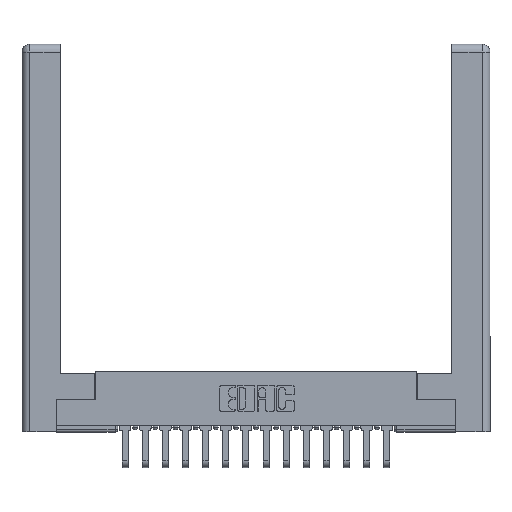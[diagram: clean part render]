
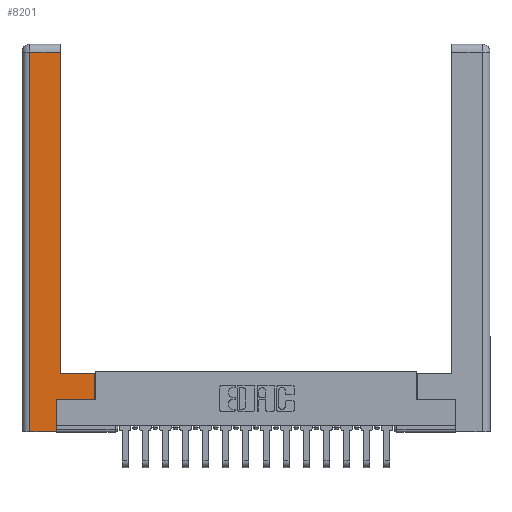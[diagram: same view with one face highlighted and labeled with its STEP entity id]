
A CAD part, top view. The second image highlights one B-rep face of the part: STEP entity #8201.
In plain terms, the highlighted planar face has unit normal (0, 0, 1).
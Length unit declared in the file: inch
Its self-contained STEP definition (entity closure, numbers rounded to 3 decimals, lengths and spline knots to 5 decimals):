
#831 = LINE ( 'NONE', #16335, #7958 ) ;
#1031 = EDGE_LOOP ( 'NONE', ( #1408, #15679, #2435, #8291, #12992, #19018, #1727, #8142 ) ) ;
#1349 = VERTEX_POINT ( 'NONE', #10223 ) ;
#1408 = ORIENTED_EDGE ( 'NONE', *, *, #2573, .T. ) ;
#1727 = ORIENTED_EDGE ( 'NONE', *, *, #9225, .T. ) ;
#1850 = EDGE_CURVE ( 'NONE', #8117, #19483, #16574, .T. ) ;
#2435 = ORIENTED_EDGE ( 'NONE', *, *, #6949, .T. ) ;
#2557 = LINE ( 'NONE', #5587, #18564 ) ;
#2573 = EDGE_CURVE ( 'NONE', #5505, #6391, #17451, .T. ) ;
#2696 = CARTESIAN_POINT ( 'NONE',  ( 0.265, 0.245, 0. ) ) ;
#4311 = CARTESIAN_POINT ( 'NONE',  ( 0., 0., 0. ) ) ;
#5319 = VERTEX_POINT ( 'NONE', #11188 ) ;
#5505 = VERTEX_POINT ( 'NONE', #19781 ) ;
#5572 = LINE ( 'NONE', #16905, #6307 ) ;
#5587 = CARTESIAN_POINT ( 'NONE',  ( 0.295, 0.45, 0. ) ) ;
#6307 = VECTOR ( 'NONE', #16801, 39.37008 ) ;
#6391 = VERTEX_POINT ( 'NONE', #8984 ) ;
#6899 = CARTESIAN_POINT ( 'NONE',  ( 0.265, 0.245, 0. ) ) ;
#6949 = EDGE_CURVE ( 'NONE', #14596, #1349, #13199, .T. ) ;
#7337 = VERTEX_POINT ( 'NONE', #15711 ) ;
#7401 = VECTOR ( 'NONE', #8657, 39.37008 ) ;
#7550 = DIRECTION ( 'NONE',  ( 0., 0., -1. ) ) ;
#7958 = VECTOR ( 'NONE', #16043, 39.37008 ) ;
#8117 = VERTEX_POINT ( 'NONE', #17798 ) ;
#8142 = ORIENTED_EDGE ( 'NONE', *, *, #8418, .T. ) ;
#8201 = ADVANCED_FACE ( 'NONE', ( #16780 ), #15169, .F. ) ;
#8291 = ORIENTED_EDGE ( 'NONE', *, *, #10828, .T. ) ;
#8418 = EDGE_CURVE ( 'NONE', #7337, #5505, #2557, .T. ) ;
#8657 = DIRECTION ( 'NONE',  ( 0., 1., 0. ) ) ;
#8984 = CARTESIAN_POINT ( 'NONE',  ( 0.295, 2.94, 0. ) ) ;
#9225 = EDGE_CURVE ( 'NONE', #5319, #7337, #14633, .T. ) ;
#9686 = EDGE_CURVE ( 'NONE', #19483, #5319, #5572, .T. ) ;
#9858 = DIRECTION ( 'NONE',  ( 0., 1., 0. ) ) ;
#9977 = DIRECTION ( 'NONE',  ( 0., 1., 0. ) ) ;
#10166 = AXIS2_PLACEMENT_3D ( 'NONE', #4311, #7550, #18402 ) ;
#10223 = CARTESIAN_POINT ( 'NONE',  ( 0.0615, 0., 0. ) ) ;
#10381 = VECTOR ( 'NONE', #9858, 39.37008 ) ;
#10700 = CARTESIAN_POINT ( 'NONE',  ( 0.0615, 2.94, 0. ) ) ;
#10828 = EDGE_CURVE ( 'NONE', #1349, #8117, #831, .T. ) ;
#11172 = DIRECTION ( 'NONE',  ( 0., -1., 0. ) ) ;
#11188 = CARTESIAN_POINT ( 'NONE',  ( 0.565, 0.245, 0. ) ) ;
#12700 = CARTESIAN_POINT ( 'NONE',  ( 0.295, 3., 0. ) ) ;
#12992 = ORIENTED_EDGE ( 'NONE', *, *, #1850, .T. ) ;
#13199 = LINE ( 'NONE', #19274, #13685 ) ;
#13685 = VECTOR ( 'NONE', #11172, 39.37008 ) ;
#14384 = VECTOR ( 'NONE', #9977, 39.37008 ) ;
#14596 = VERTEX_POINT ( 'NONE', #19145 ) ;
#14633 = LINE ( 'NONE', #17675, #14384 ) ;
#15169 = PLANE ( 'NONE',  #10166 ) ;
#15363 = EDGE_CURVE ( 'NONE', #6391, #14596, #16886, .T. ) ;
#15679 = ORIENTED_EDGE ( 'NONE', *, *, #15363, .T. ) ;
#15711 = CARTESIAN_POINT ( 'NONE',  ( 0.565, 0.45, 0. ) ) ;
#16043 = DIRECTION ( 'NONE',  ( 1., 0., 0. ) ) ;
#16335 = CARTESIAN_POINT ( 'NONE',  ( 0.265, 0., 0. ) ) ;
#16471 = VECTOR ( 'NONE', #18507, 39.37008 ) ;
#16574 = LINE ( 'NONE', #2696, #7401 ) ;
#16780 = FACE_OUTER_BOUND ( 'NONE', #1031, .T. ) ;
#16801 = DIRECTION ( 'NONE',  ( 1., 0., 0. ) ) ;
#16886 = LINE ( 'NONE', #10700, #16471 ) ;
#16905 = CARTESIAN_POINT ( 'NONE',  ( 0.565, 0.245, 0. ) ) ;
#17451 = LINE ( 'NONE', #12700, #10381 ) ;
#17675 = CARTESIAN_POINT ( 'NONE',  ( 0.565, 0.45, 0. ) ) ;
#17798 = CARTESIAN_POINT ( 'NONE',  ( 0.265, 0., 0. ) ) ;
#18402 = DIRECTION ( 'NONE',  ( -1., 0., 0. ) ) ;
#18507 = DIRECTION ( 'NONE',  ( -1., 0., 0. ) ) ;
#18564 = VECTOR ( 'NONE', #19493, 39.37008 ) ;
#19018 = ORIENTED_EDGE ( 'NONE', *, *, #9686, .T. ) ;
#19145 = CARTESIAN_POINT ( 'NONE',  ( 0.0615, 2.94, 0. ) ) ;
#19274 = CARTESIAN_POINT ( 'NONE',  ( 0.0615, 0., 0. ) ) ;
#19483 = VERTEX_POINT ( 'NONE', #6899 ) ;
#19493 = DIRECTION ( 'NONE',  ( -1., 0., 0. ) ) ;
#19781 = CARTESIAN_POINT ( 'NONE',  ( 0.295, 0.45, 0. ) ) ;
